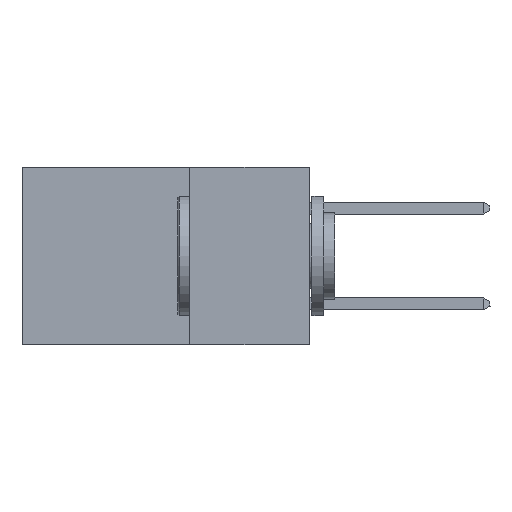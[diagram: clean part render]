
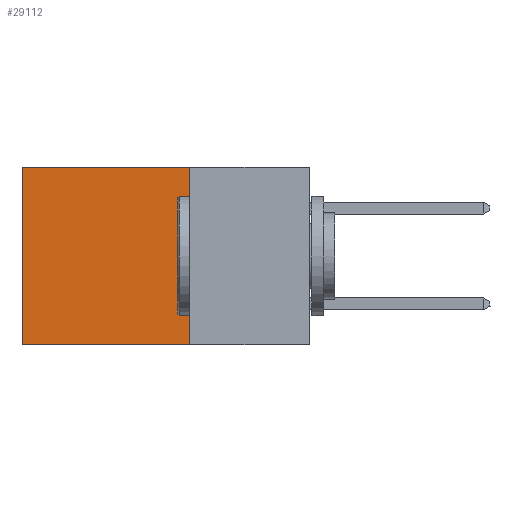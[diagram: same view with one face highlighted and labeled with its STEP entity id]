
A CAD part, left-side view. The second image highlights one B-rep face of the part: STEP entity #29112.
In plain terms, the highlighted planar face has unit normal (-1, 0, 0).
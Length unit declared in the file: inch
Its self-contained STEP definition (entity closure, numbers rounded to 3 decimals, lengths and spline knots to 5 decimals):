
#1074 = EDGE_CURVE ( 'NONE', #25376, #27793, #16898, .T. ) ;
#1762 = VECTOR ( 'NONE', #11215, 39.37008 ) ;
#2292 = DIRECTION ( 'NONE',  ( 0., 1., 0. ) ) ;
#2735 = CARTESIAN_POINT ( 'NONE',  ( 0.2875, 0.6, -0.37 ) ) ;
#3103 = FACE_OUTER_BOUND ( 'NONE', #17758, .T. ) ;
#3880 = DIRECTION ( 'NONE',  ( 0., 0., -1. ) ) ;
#5479 = CARTESIAN_POINT ( 'NONE',  ( 0.2875, 0.25, 0. ) ) ;
#6050 = CARTESIAN_POINT ( 'NONE',  ( 0.2875, 0.25, 0. ) ) ;
#6487 = DIRECTION ( 'NONE',  ( 0., 0., -1. ) ) ;
#7646 = VERTEX_POINT ( 'NONE', #6050 ) ;
#8895 = CARTESIAN_POINT ( 'NONE',  ( 0.2875, 0.25, -0.37 ) ) ;
#9060 = EDGE_CURVE ( 'NONE', #7646, #22812, #17526, .T. ) ;
#9381 = EDGE_CURVE ( 'NONE', #7646, #25376, #29676, .T. ) ;
#10726 = CARTESIAN_POINT ( 'NONE',  ( 0.2875, 0.25, 0. ) ) ;
#11105 = AXIS2_PLACEMENT_3D ( 'NONE', #10726, #20276, #6487 ) ;
#11215 = DIRECTION ( 'NONE',  ( 0., 1., 0. ) ) ;
#11531 = VECTOR ( 'NONE', #3880, 39.37008 ) ;
#12473 = EDGE_CURVE ( 'NONE', #22812, #27793, #28736, .T. ) ;
#13603 = ORIENTED_EDGE ( 'NONE', *, *, #9060, .T. ) ;
#15453 = ORIENTED_EDGE ( 'NONE', *, *, #1074, .F. ) ;
#16769 = ORIENTED_EDGE ( 'NONE', *, *, #9381, .F. ) ;
#16808 = VECTOR ( 'NONE', #2292, 39.37008 ) ;
#16898 = LINE ( 'NONE', #8895, #1762 ) ;
#16971 = CARTESIAN_POINT ( 'NONE',  ( 0.2875, 0.6, 0. ) ) ;
#17501 = VECTOR ( 'NONE', #19481, 39.37008 ) ;
#17526 = LINE ( 'NONE', #27528, #16808 ) ;
#17758 = EDGE_LOOP ( 'NONE', ( #27630, #15453, #16769, #13603 ) ) ;
#19481 = DIRECTION ( 'NONE',  ( 0., 0., -1. ) ) ;
#20151 = CARTESIAN_POINT ( 'NONE',  ( 0.2875, 0.25, -0.37 ) ) ;
#20276 = DIRECTION ( 'NONE',  ( 1., 0., 0. ) ) ;
#22496 = CARTESIAN_POINT ( 'NONE',  ( 0.2875, 0.6, 0. ) ) ;
#22812 = VERTEX_POINT ( 'NONE', #16971 ) ;
#24698 = PLANE ( 'NONE',  #11105 ) ;
#25376 = VERTEX_POINT ( 'NONE', #20151 ) ;
#27528 = CARTESIAN_POINT ( 'NONE',  ( 0.2875, 0.25, 0. ) ) ;
#27630 = ORIENTED_EDGE ( 'NONE', *, *, #12473, .T. ) ;
#27793 = VERTEX_POINT ( 'NONE', #2735 ) ;
#28736 = LINE ( 'NONE', #22496, #11531 ) ;
#29112 = ADVANCED_FACE ( 'NONE', ( #3103 ), #24698, .F. ) ;
#29676 = LINE ( 'NONE', #5479, #17501 ) ;
